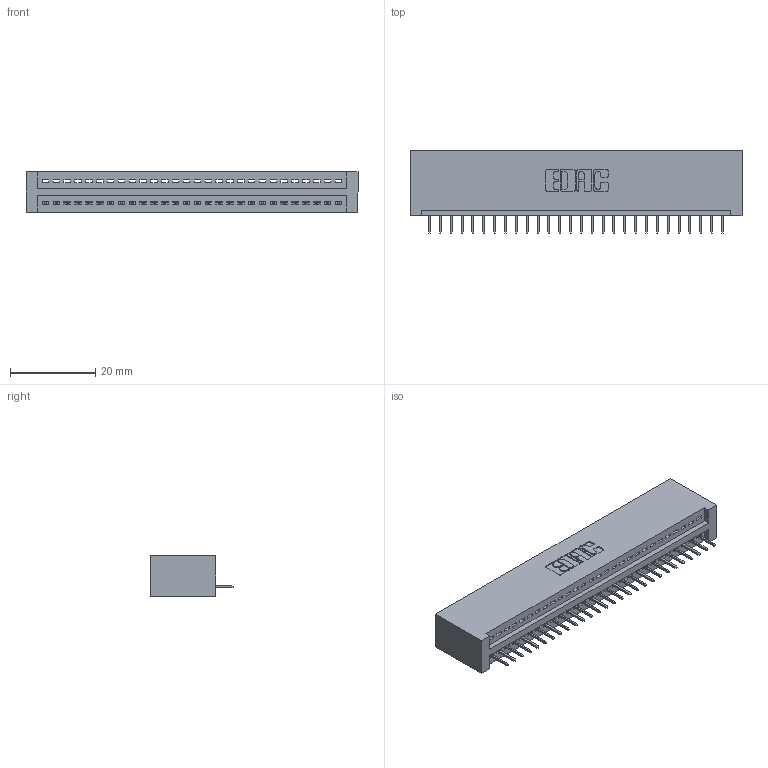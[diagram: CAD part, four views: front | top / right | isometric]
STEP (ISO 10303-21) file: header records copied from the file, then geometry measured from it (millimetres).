
FILE_DESCRIPTION (( 'STEP AP203' ), '1' );
FILE_NAME ('395-028-524-101.STEP', '2019-10-19T03:39:06', ( '' ), ( '' ), 'SwSTEP 2.0', 'SolidWorks 2016', '' );
FILE_SCHEMA (( 'CONFIG_CONTROL_DESIGN' ));
Length unit declared in the file: inch
Products named in the file (3): 395-028-524-101; 345-292-001_345-293-124; 345 Part_No Mounting Lugs
Assembly tree (29 placements, depth 2):
  395-028-524-101
    345 Part_No Mounting Lugs
    345-292-001_345-293-124  x28
Bounding box: 77.72 x 19.35 x 9.4 mm (x, y, z)
Volume: 7741.4 mm3; surface area: 9933.8 mm2
Topology: 29 solids, 29 shells, 1854 faces, 5357 edges, 3458 vertices
Faces by surface type: plane 1364, cylinder 490
Entity records: 22755 total; most frequent: CARTESIAN_POINT 3948, ORIENTED_EDGE 3910, DIRECTION 3463, EDGE_CURVE 1955, VECTOR 1723, LINE 1723, VERTEX_POINT 1298, AXIS2_PLACEMENT_3D 870
